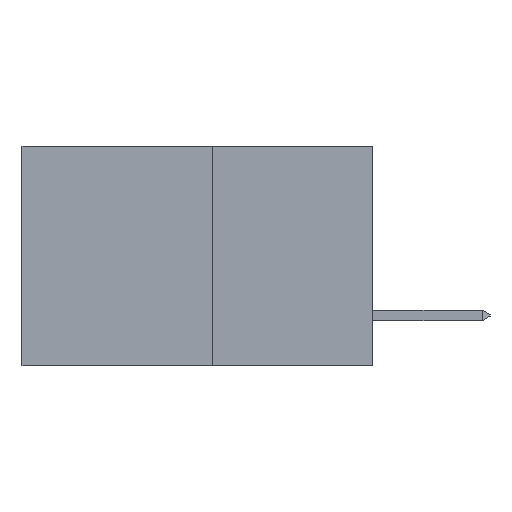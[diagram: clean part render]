
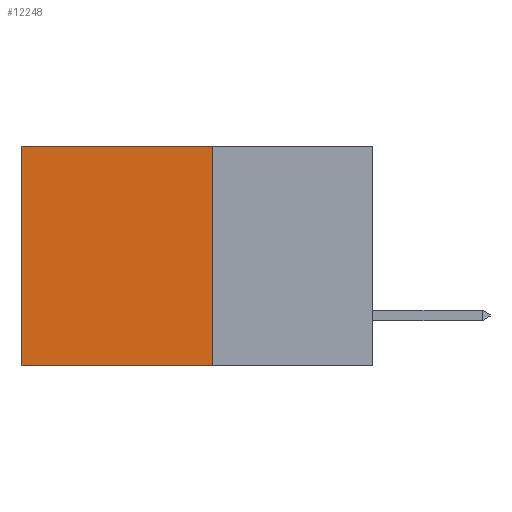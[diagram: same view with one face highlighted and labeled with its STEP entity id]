
A CAD part, left-side view. The second image highlights one B-rep face of the part: STEP entity #12248.
In plain terms, the highlighted planar face has unit normal (-1, 0, 0).
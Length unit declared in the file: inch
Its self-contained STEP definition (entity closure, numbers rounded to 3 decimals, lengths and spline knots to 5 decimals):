
#43 = CARTESIAN_POINT ( 'NONE',  ( 0.277, 0.59, -0.37 ) ) ;
#540 = ORIENTED_EDGE ( 'NONE', *, *, #14676, .T. ) ;
#591 = DIRECTION ( 'NONE',  ( 0., 1., 0. ) ) ;
#1837 = PLANE ( 'NONE',  #5480 ) ;
#2148 = EDGE_LOOP ( 'NONE', ( #17718, #3599, #7925, #540 ) ) ;
#2853 = VERTEX_POINT ( 'NONE', #43 ) ;
#3164 = FACE_OUTER_BOUND ( 'NONE', #2148, .T. ) ;
#3327 = CARTESIAN_POINT ( 'NONE',  ( 0.277, 0.27, 0. ) ) ;
#3336 = DIRECTION ( 'NONE',  ( 1., 0., 0. ) ) ;
#3446 = DIRECTION ( 'NONE',  ( 0., 1., 0. ) ) ;
#3548 = LINE ( 'NONE', #18209, #18540 ) ;
#3599 = ORIENTED_EDGE ( 'NONE', *, *, #7248, .F. ) ;
#4571 = VERTEX_POINT ( 'NONE', #11636 ) ;
#5199 = VERTEX_POINT ( 'NONE', #3327 ) ;
#5480 = AXIS2_PLACEMENT_3D ( 'NONE', #12096, #3336, #13615 ) ;
#6163 = CARTESIAN_POINT ( 'NONE',  ( 0.277, 0.27, -0.37 ) ) ;
#6738 = LINE ( 'NONE', #6163, #15083 ) ;
#6884 = VECTOR ( 'NONE', #18467, 39.37008 ) ;
#7248 = EDGE_CURVE ( 'NONE', #11418, #2853, #6738, .T. ) ;
#7925 = ORIENTED_EDGE ( 'NONE', *, *, #16120, .F. ) ;
#8793 = CARTESIAN_POINT ( 'NONE',  ( 0.277, 0.27, -0.37 ) ) ;
#11418 = VERTEX_POINT ( 'NONE', #8793 ) ;
#11636 = CARTESIAN_POINT ( 'NONE',  ( 0.277, 0.59, 0. ) ) ;
#11991 = VECTOR ( 'NONE', #591, 39.37008 ) ;
#12096 = CARTESIAN_POINT ( 'NONE',  ( 0.277, 0.27, -0.37 ) ) ;
#12248 = ADVANCED_FACE ( 'NONE', ( #3164 ), #1837, .F. ) ;
#13615 = DIRECTION ( 'NONE',  ( 0., 0., -1. ) ) ;
#14676 = EDGE_CURVE ( 'NONE', #5199, #4571, #15905, .T. ) ;
#14782 = LINE ( 'NONE', #17123, #6884 ) ;
#15083 = VECTOR ( 'NONE', #3446, 39.37008 ) ;
#15600 = DIRECTION ( 'NONE',  ( 0., 0., -1. ) ) ;
#15905 = LINE ( 'NONE', #18093, #11991 ) ;
#16120 = EDGE_CURVE ( 'NONE', #5199, #11418, #14782, .T. ) ;
#17123 = CARTESIAN_POINT ( 'NONE',  ( 0.277, 0.27, -0.37 ) ) ;
#17585 = EDGE_CURVE ( 'NONE', #4571, #2853, #3548, .T. ) ;
#17718 = ORIENTED_EDGE ( 'NONE', *, *, #17585, .T. ) ;
#18093 = CARTESIAN_POINT ( 'NONE',  ( 0.277, 0.27, 0. ) ) ;
#18209 = CARTESIAN_POINT ( 'NONE',  ( 0.277, 0.59, -0.37 ) ) ;
#18467 = DIRECTION ( 'NONE',  ( 0., 0., -1. ) ) ;
#18540 = VECTOR ( 'NONE', #15600, 39.37008 ) ;
